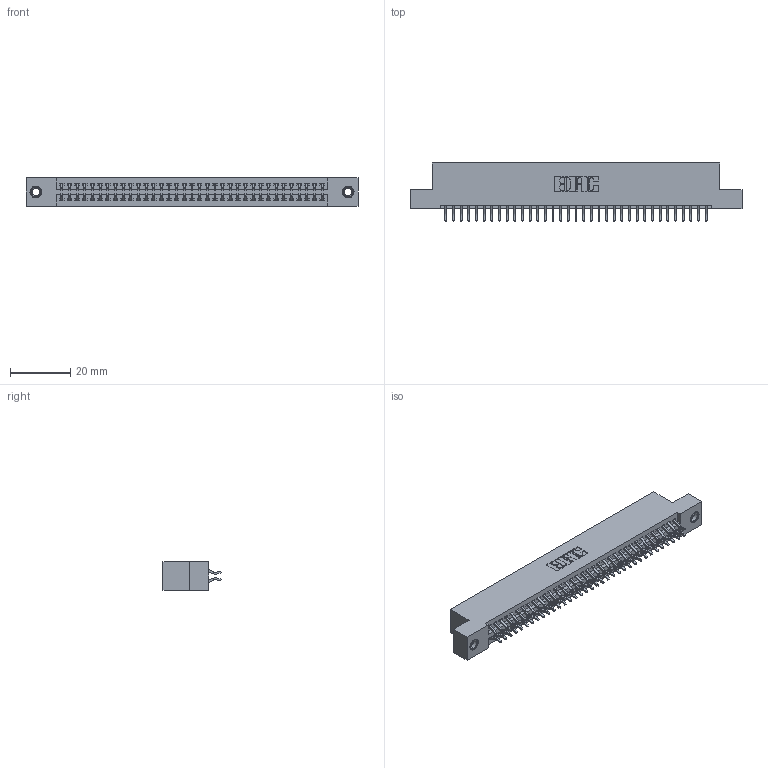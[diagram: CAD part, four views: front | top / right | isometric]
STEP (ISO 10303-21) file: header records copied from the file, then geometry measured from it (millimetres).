
FILE_DESCRIPTION (( 'STEP AP203' ), '1' );
FILE_NAME ('395-070-556-207.STEP', '2019-10-24T10:57:27', ( '' ), ( '' ), 'SwSTEP 2.0', 'SolidWorks 2016', '' );
FILE_SCHEMA (( 'CONFIG_CONTROL_DESIGN' ));
Length unit declared in the file: inch
Products named in the file (4): 345 Part_Flush Mounting Lugs - 0.156 Dia-TI; 345-292-001_556 Tail; 345-250-001_345-250-005-103; 395-070-556-207
Assembly tree (73 placements, depth 2):
  395-070-556-207
    345 Part_Flush Mounting Lugs - 0.156 Dia-TI
    345-292-001_556 Tail  x70
    345-250-001_345-250-005-103  x2
Bounding box: 110.11 x 19.24 x 9.4 mm (x, y, z)
Volume: 10614.8 mm3; surface area: 15521.5 mm2
Topology: 73 solids, 73 shells, 4106 faces, 12167 edges, 8010 vertices
Faces by surface type: plane 2702, cylinder 1388, cone 12, torus 4
Entity records: 29810 total; most frequent: CARTESIAN_POINT 4999, ORIENTED_EDGE 4914, DIRECTION 4431, EDGE_CURVE 2457, LINE 2157, VECTOR 2157, VERTEX_POINT 1632, AXIS2_PLACEMENT_3D 1137
